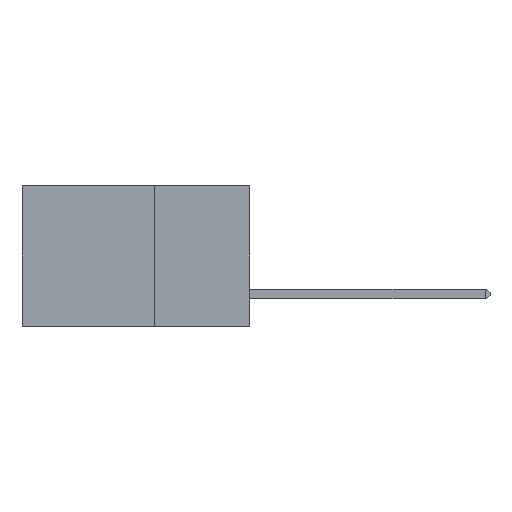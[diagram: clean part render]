
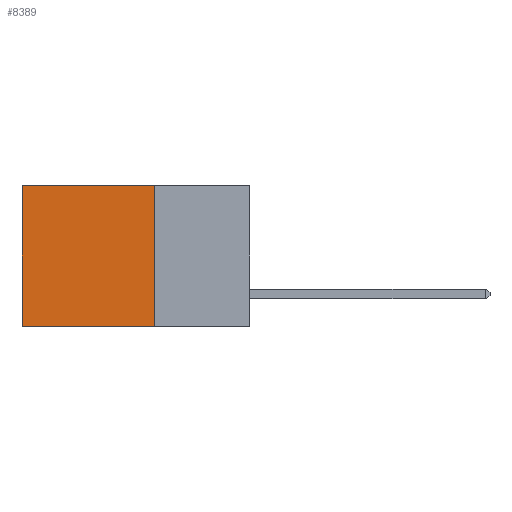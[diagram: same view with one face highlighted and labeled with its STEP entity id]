
A CAD part, left-side view. The second image highlights one B-rep face of the part: STEP entity #8389.
In plain terms, the highlighted planar face has unit normal (-1, 0, 0).
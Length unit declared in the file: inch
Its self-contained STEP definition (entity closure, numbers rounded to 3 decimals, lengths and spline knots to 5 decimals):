
#309 = EDGE_CURVE ( 'NONE', #8987, #18015, #9126, .T. ) ;
#2030 = VERTEX_POINT ( 'NONE', #15733 ) ;
#2421 = LINE ( 'NONE', #7935, #8025 ) ;
#4902 = DIRECTION ( 'NONE',  ( 0., 0., -1. ) ) ;
#4955 = LINE ( 'NONE', #23955, #6678 ) ;
#5602 = EDGE_CURVE ( 'NONE', #29678, #18015, #2421, .T. ) ;
#6509 = DIRECTION ( 'NONE',  ( 1., 0., 0. ) ) ;
#6678 = VECTOR ( 'NONE', #4902, 39.37008 ) ;
#7812 = DIRECTION ( 'NONE',  ( 0., 1., 0. ) ) ;
#7935 = CARTESIAN_POINT ( 'NONE',  ( 0.2875, 0.25, -0.37 ) ) ;
#8025 = VECTOR ( 'NONE', #7812, 39.37008 ) ;
#8389 = ADVANCED_FACE ( 'NONE', ( #16309 ), #11921, .F. ) ;
#8987 = VERTEX_POINT ( 'NONE', #34290 ) ;
#9126 = LINE ( 'NONE', #34371, #21903 ) ;
#10032 = DIRECTION ( 'NONE',  ( 0., 0., -1. ) ) ;
#11921 = PLANE ( 'NONE',  #22015 ) ;
#12272 = ORIENTED_EDGE ( 'NONE', *, *, #309, .T. ) ;
#12283 = EDGE_CURVE ( 'NONE', #2030, #29678, #4955, .T. ) ;
#12514 = CARTESIAN_POINT ( 'NONE',  ( 0.2875, 0.6, -0.37 ) ) ;
#14180 = EDGE_CURVE ( 'NONE', #2030, #8987, #35017, .T. ) ;
#15733 = CARTESIAN_POINT ( 'NONE',  ( 0.2875, 0.25, 0. ) ) ;
#15804 = CARTESIAN_POINT ( 'NONE',  ( 0.2875, 0.25, -0.37 ) ) ;
#16309 = FACE_OUTER_BOUND ( 'NONE', #27695, .T. ) ;
#18015 = VERTEX_POINT ( 'NONE', #12514 ) ;
#18261 = ORIENTED_EDGE ( 'NONE', *, *, #14180, .T. ) ;
#19212 = DIRECTION ( 'NONE',  ( 0., 1., 0. ) ) ;
#20071 = CARTESIAN_POINT ( 'NONE',  ( 0.2875, 0.25, 0. ) ) ;
#20586 = VECTOR ( 'NONE', #19212, 39.37008 ) ;
#21903 = VECTOR ( 'NONE', #10032, 39.37008 ) ;
#22015 = AXIS2_PLACEMENT_3D ( 'NONE', #20071, #6509, #25514 ) ;
#22096 = ORIENTED_EDGE ( 'NONE', *, *, #5602, .F. ) ;
#23955 = CARTESIAN_POINT ( 'NONE',  ( 0.2875, 0.25, 0. ) ) ;
#24195 = ORIENTED_EDGE ( 'NONE', *, *, #12283, .F. ) ;
#25514 = DIRECTION ( 'NONE',  ( 0., 0., -1. ) ) ;
#27261 = CARTESIAN_POINT ( 'NONE',  ( 0.2875, 0.25, 0. ) ) ;
#27695 = EDGE_LOOP ( 'NONE', ( #12272, #22096, #24195, #18261 ) ) ;
#29678 = VERTEX_POINT ( 'NONE', #15804 ) ;
#34290 = CARTESIAN_POINT ( 'NONE',  ( 0.2875, 0.6, 0. ) ) ;
#34371 = CARTESIAN_POINT ( 'NONE',  ( 0.2875, 0.6, 0. ) ) ;
#35017 = LINE ( 'NONE', #27261, #20586 ) ;
